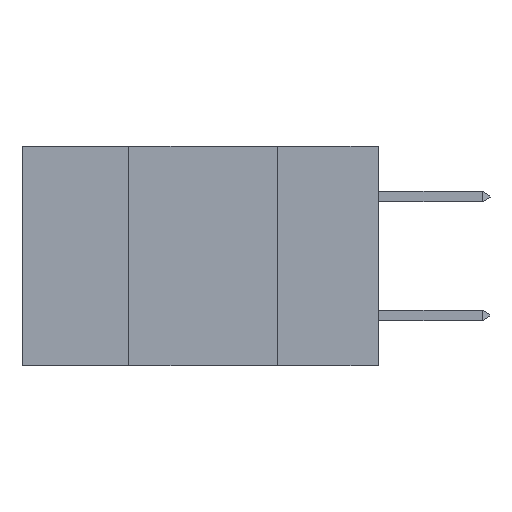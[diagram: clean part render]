
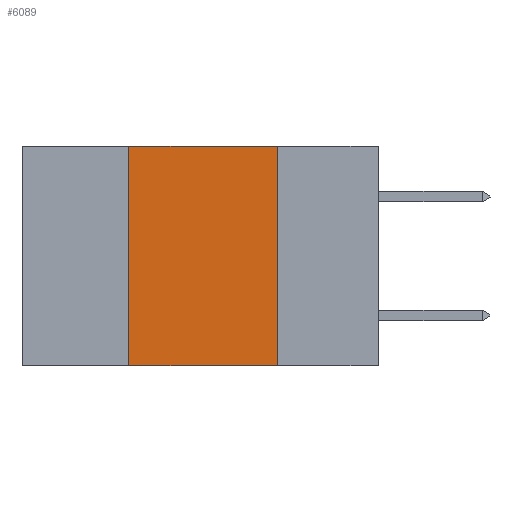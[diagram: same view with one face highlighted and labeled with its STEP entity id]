
A CAD part, left-side view. The second image highlights one B-rep face of the part: STEP entity #6089.
In plain terms, the highlighted planar face has unit normal (-1, 0, 0).
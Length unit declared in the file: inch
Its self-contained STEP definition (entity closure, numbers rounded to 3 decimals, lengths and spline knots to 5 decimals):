
#561 = CARTESIAN_POINT ( 'NONE',  ( 0., 0.6, -0.37 ) ) ;
#2132 = ORIENTED_EDGE ( 'NONE', *, *, #29115, .F. ) ;
#4706 = VECTOR ( 'NONE', #30508, 39.37008 ) ;
#4717 = CARTESIAN_POINT ( 'NONE',  ( 0., 0.17, 0. ) ) ;
#5253 = CARTESIAN_POINT ( 'NONE',  ( 0., 0.6, 0. ) ) ;
#5318 = EDGE_LOOP ( 'NONE', ( #14652, #31872, #2132, #9227 ) ) ;
#5459 = CARTESIAN_POINT ( 'NONE',  ( 0., 0.42, 0. ) ) ;
#6089 = ADVANCED_FACE ( 'NONE', ( #13136 ), #13341, .F. ) ;
#8582 = VERTEX_POINT ( 'NONE', #32550 ) ;
#8991 = DIRECTION ( 'NONE',  ( 1., 0., 0. ) ) ;
#9227 = ORIENTED_EDGE ( 'NONE', *, *, #27956, .T. ) ;
#9270 = VERTEX_POINT ( 'NONE', #4717 ) ;
#9422 = AXIS2_PLACEMENT_3D ( 'NONE', #28057, #8991, #27435 ) ;
#12792 = VECTOR ( 'NONE', #13079, 39.37008 ) ;
#13079 = DIRECTION ( 'NONE',  ( 0., 0., -1. ) ) ;
#13136 = FACE_OUTER_BOUND ( 'NONE', #5318, .T. ) ;
#13341 = PLANE ( 'NONE',  #9422 ) ;
#14652 = ORIENTED_EDGE ( 'NONE', *, *, #19460, .F. ) ;
#15804 = DIRECTION ( 'NONE',  ( 0., -1., 0. ) ) ;
#15975 = LINE ( 'NONE', #19944, #21883 ) ;
#16402 = EDGE_CURVE ( 'NONE', #16779, #9270, #24933, .T. ) ;
#16779 = VERTEX_POINT ( 'NONE', #5459 ) ;
#18021 = LINE ( 'NONE', #561, #23957 ) ;
#19460 = EDGE_CURVE ( 'NONE', #9270, #22454, #26280, .T. ) ;
#19944 = CARTESIAN_POINT ( 'NONE',  ( 0., 0.42, 0. ) ) ;
#21883 = VECTOR ( 'NONE', #25046, 39.37008 ) ;
#22454 = VERTEX_POINT ( 'NONE', #32149 ) ;
#23957 = VECTOR ( 'NONE', #15804, 39.37008 ) ;
#24933 = LINE ( 'NONE', #5253, #4706 ) ;
#25046 = DIRECTION ( 'NONE',  ( 0., 0., 1. ) ) ;
#25596 = CARTESIAN_POINT ( 'NONE',  ( 0., 0.17, 0. ) ) ;
#26280 = LINE ( 'NONE', #25596, #12792 ) ;
#27435 = DIRECTION ( 'NONE',  ( 0., 0., -1. ) ) ;
#27956 = EDGE_CURVE ( 'NONE', #8582, #22454, #18021, .T. ) ;
#28057 = CARTESIAN_POINT ( 'NONE',  ( 0., 0.6, 0. ) ) ;
#29115 = EDGE_CURVE ( 'NONE', #8582, #16779, #15975, .T. ) ;
#30508 = DIRECTION ( 'NONE',  ( 0., -1., 0. ) ) ;
#31872 = ORIENTED_EDGE ( 'NONE', *, *, #16402, .F. ) ;
#32149 = CARTESIAN_POINT ( 'NONE',  ( 0., 0.17, -0.37 ) ) ;
#32550 = CARTESIAN_POINT ( 'NONE',  ( 0., 0.42, -0.37 ) ) ;
